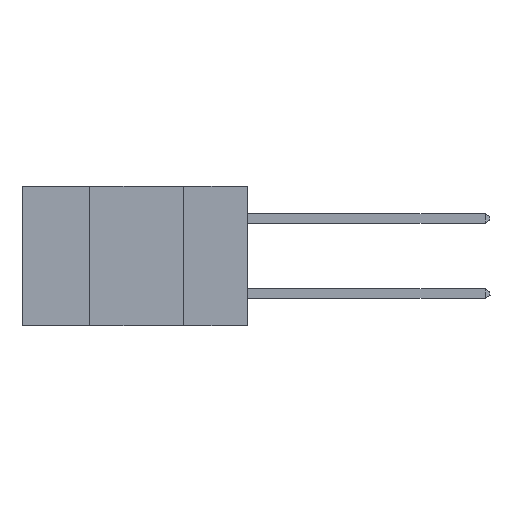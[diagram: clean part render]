
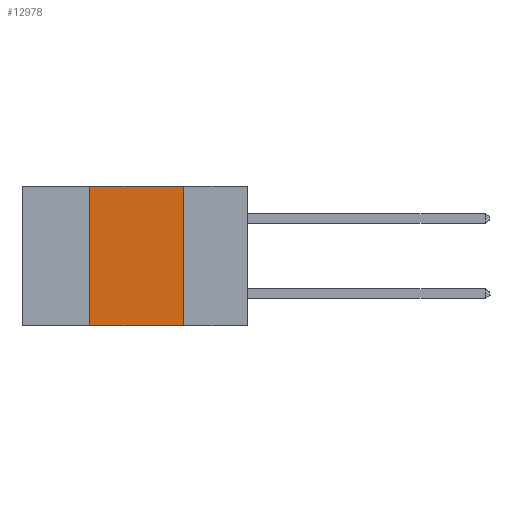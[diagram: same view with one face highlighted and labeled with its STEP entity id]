
A CAD part, left-side view. The second image highlights one B-rep face of the part: STEP entity #12978.
In plain terms, the highlighted planar face has unit normal (-1, 0, 0).
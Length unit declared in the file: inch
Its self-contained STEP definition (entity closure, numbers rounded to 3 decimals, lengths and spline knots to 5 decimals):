
#187 = EDGE_CURVE ( 'NONE', #4611, #18990, #1641, .T. ) ;
#828 = CARTESIAN_POINT ( 'NONE',  ( 0., 0.42, 0. ) ) ;
#869 = ORIENTED_EDGE ( 'NONE', *, *, #11180, .F. ) ;
#1356 = DIRECTION ( 'NONE',  ( 0., 0., -1. ) ) ;
#1641 = LINE ( 'NONE', #3294, #27207 ) ;
#1652 = VECTOR ( 'NONE', #27958, 39.37008 ) ;
#2054 = VERTEX_POINT ( 'NONE', #8824 ) ;
#2541 = LINE ( 'NONE', #828, #9454 ) ;
#3294 = CARTESIAN_POINT ( 'NONE',  ( 0., 0.17, 0. ) ) ;
#4611 = VERTEX_POINT ( 'NONE', #22075 ) ;
#5651 = AXIS2_PLACEMENT_3D ( 'NONE', #11590, #6458, #1356 ) ;
#5843 = LINE ( 'NONE', #20167, #26380 ) ;
#6458 = DIRECTION ( 'NONE',  ( 1., 0., 0. ) ) ;
#8256 = FACE_OUTER_BOUND ( 'NONE', #18417, .T. ) ;
#8304 = ORIENTED_EDGE ( 'NONE', *, *, #187, .F. ) ;
#8354 = DIRECTION ( 'NONE',  ( 0., 0., -1. ) ) ;
#8824 = CARTESIAN_POINT ( 'NONE',  ( 0., 0.42, 0. ) ) ;
#9416 = EDGE_CURVE ( 'NONE', #29848, #18990, #31483, .T. ) ;
#9454 = VECTOR ( 'NONE', #23145, 39.37008 ) ;
#10992 = CARTESIAN_POINT ( 'NONE',  ( 0., 0.6, -0.37 ) ) ;
#11180 = EDGE_CURVE ( 'NONE', #2054, #4611, #5843, .T. ) ;
#11318 = CARTESIAN_POINT ( 'NONE',  ( 0., 0.42, -0.37 ) ) ;
#11590 = CARTESIAN_POINT ( 'NONE',  ( 0., 0.6, 0. ) ) ;
#12978 = ADVANCED_FACE ( 'NONE', ( #8256 ), #31458, .F. ) ;
#15781 = EDGE_CURVE ( 'NONE', #29848, #2054, #2541, .T. ) ;
#17250 = DIRECTION ( 'NONE',  ( 0., -1., 0. ) ) ;
#18417 = EDGE_LOOP ( 'NONE', ( #8304, #869, #28650, #27512 ) ) ;
#18990 = VERTEX_POINT ( 'NONE', #30519 ) ;
#20167 = CARTESIAN_POINT ( 'NONE',  ( 0., 0.6, 0. ) ) ;
#22075 = CARTESIAN_POINT ( 'NONE',  ( 0., 0.17, 0. ) ) ;
#23145 = DIRECTION ( 'NONE',  ( 0., 0., 1. ) ) ;
#26380 = VECTOR ( 'NONE', #17250, 39.37008 ) ;
#27207 = VECTOR ( 'NONE', #8354, 39.37008 ) ;
#27512 = ORIENTED_EDGE ( 'NONE', *, *, #9416, .T. ) ;
#27958 = DIRECTION ( 'NONE',  ( 0., -1., 0. ) ) ;
#28650 = ORIENTED_EDGE ( 'NONE', *, *, #15781, .F. ) ;
#29848 = VERTEX_POINT ( 'NONE', #11318 ) ;
#30519 = CARTESIAN_POINT ( 'NONE',  ( 0., 0.17, -0.37 ) ) ;
#31458 = PLANE ( 'NONE',  #5651 ) ;
#31483 = LINE ( 'NONE', #10992, #1652 ) ;
